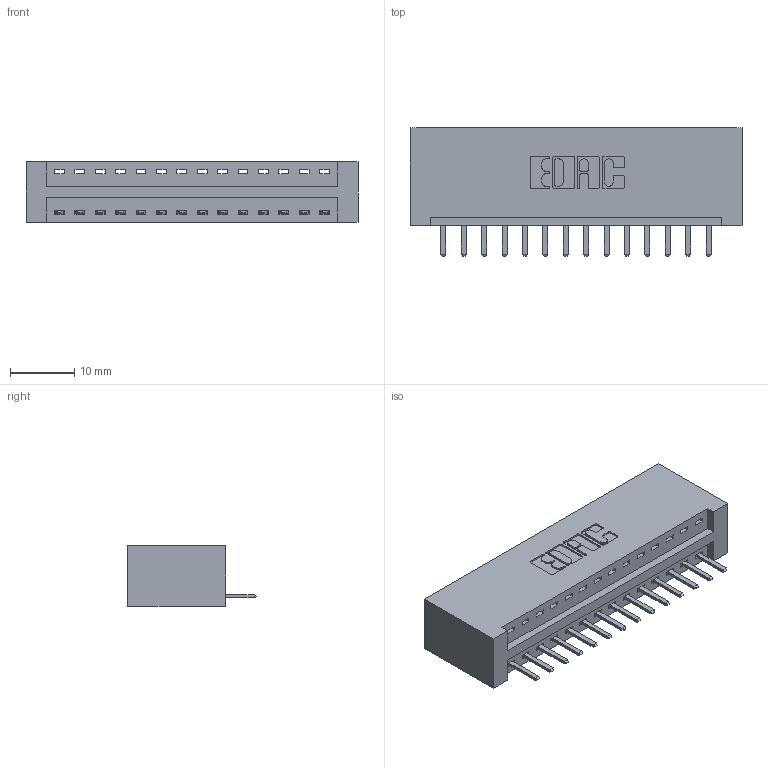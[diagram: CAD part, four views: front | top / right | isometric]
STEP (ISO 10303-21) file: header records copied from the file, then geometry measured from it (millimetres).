
FILE_DESCRIPTION (( 'STEP AP203' ), '1' );
FILE_NAME ('346-014-520-101.STEP', '2022-05-05T05:38:07', ( '' ), ( '' ), 'SwSTEP 2.0', 'SolidWorks 2020', '' );
FILE_SCHEMA (( 'CONFIG_CONTROL_DESIGN' ));
Length unit declared in the file: inch
Products named in the file (3): 346-014-520-101; 346 Part_No Mounting Lugs; 345-292-001_345-293-120
Assembly tree (15 placements, depth 2):
  346-014-520-101
    346 Part_No Mounting Lugs
    345-292-001_345-293-120  x14
Bounding box: 51.69 x 20.02 x 9.4 mm (x, y, z)
Volume: 5264 mm3; surface area: 6217.9 mm2
Topology: 15 solids, 15 shells, 982 faces, 2881 edges, 1882 vertices
Faces by surface type: plane 660, cylinder 322
Entity records: 12295 total; most frequent: CARTESIAN_POINT 2134, ORIENTED_EDGE 2070, DIRECTION 1899, EDGE_CURVE 1035, VECTOR 851, LINE 851, VERTEX_POINT 686, AXIS2_PLACEMENT_3D 524
